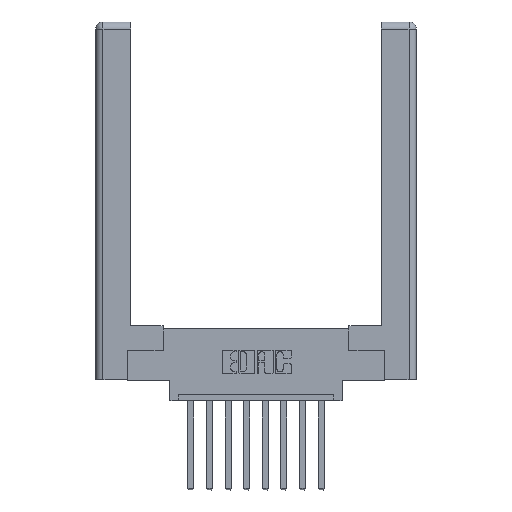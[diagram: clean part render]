
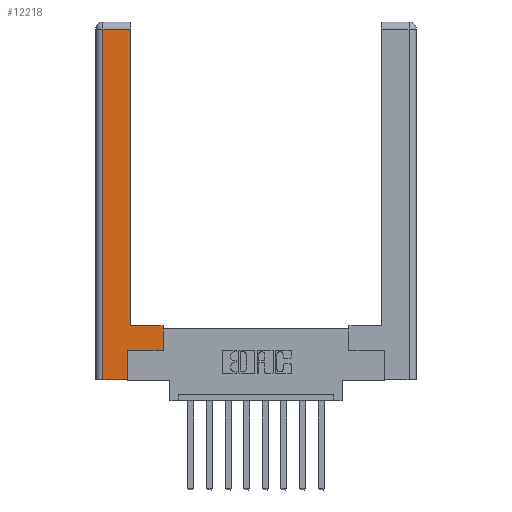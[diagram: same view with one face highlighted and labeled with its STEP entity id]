
A CAD part, top view. The second image highlights one B-rep face of the part: STEP entity #12218.
In plain terms, the highlighted planar face has unit normal (0, 0, 1).
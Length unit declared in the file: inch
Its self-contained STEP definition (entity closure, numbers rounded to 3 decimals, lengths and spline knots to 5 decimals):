
#433 = VECTOR ( 'NONE', #1633, 39.37008 ) ;
#869 = CARTESIAN_POINT ( 'NONE',  ( 0.0615, 0., 0. ) ) ;
#966 = EDGE_CURVE ( 'NONE', #11788, #7582, #6455, .T. ) ;
#1075 = VERTEX_POINT ( 'NONE', #1980 ) ;
#1281 = ORIENTED_EDGE ( 'NONE', *, *, #966, .T. ) ;
#1303 = LINE ( 'NONE', #11861, #8903 ) ;
#1392 = ORIENTED_EDGE ( 'NONE', *, *, #4505, .T. ) ;
#1480 = VERTEX_POINT ( 'NONE', #1637 ) ;
#1566 = DIRECTION ( 'NONE',  ( 0., 0., -1. ) ) ;
#1633 = DIRECTION ( 'NONE',  ( 0., 1., 0. ) ) ;
#1637 = CARTESIAN_POINT ( 'NONE',  ( 0.265, 0., 0. ) ) ;
#1784 = CARTESIAN_POINT ( 'NONE',  ( 0.0615, 2.94, 0. ) ) ;
#1980 = CARTESIAN_POINT ( 'NONE',  ( 0.295, 2.94, 0. ) ) ;
#1983 = CARTESIAN_POINT ( 'NONE',  ( 0.0615, 2.94, 0. ) ) ;
#2356 = VECTOR ( 'NONE', #12148, 39.37008 ) ;
#2391 = VECTOR ( 'NONE', #6361, 39.37008 ) ;
#3128 = ORIENTED_EDGE ( 'NONE', *, *, #3938, .T. ) ;
#3325 = CARTESIAN_POINT ( 'NONE',  ( 0.0615, 0., 0. ) ) ;
#3398 = EDGE_CURVE ( 'NONE', #7102, #9427, #4994, .T. ) ;
#3892 = EDGE_LOOP ( 'NONE', ( #7756, #9481, #7665, #5040, #1392, #8827, #1281, #3128 ) ) ;
#3938 = EDGE_CURVE ( 'NONE', #7582, #7434, #1303, .T. ) ;
#4505 = EDGE_CURVE ( 'NONE', #1480, #7061, #8411, .T. ) ;
#4525 = VECTOR ( 'NONE', #9711, 39.37008 ) ;
#4555 = EDGE_CURVE ( 'NONE', #7434, #1075, #5732, .T. ) ;
#4728 = LINE ( 'NONE', #1784, #4525 ) ;
#4894 = EDGE_CURVE ( 'NONE', #7061, #11788, #6653, .T. ) ;
#4994 = LINE ( 'NONE', #3325, #2391 ) ;
#5040 = ORIENTED_EDGE ( 'NONE', *, *, #11022, .T. ) ;
#5441 = CARTESIAN_POINT ( 'NONE',  ( 0.565, 0.245, 0. ) ) ;
#5732 = LINE ( 'NONE', #6259, #2356 ) ;
#5892 = DIRECTION ( 'NONE',  ( 1., 0., 0. ) ) ;
#6081 = EDGE_CURVE ( 'NONE', #1075, #7102, #4728, .T. ) ;
#6259 = CARTESIAN_POINT ( 'NONE',  ( 0.295, 3., 0. ) ) ;
#6361 = DIRECTION ( 'NONE',  ( 0., -1., 0. ) ) ;
#6382 = CARTESIAN_POINT ( 'NONE',  ( 0.265, 0., 0. ) ) ;
#6455 = LINE ( 'NONE', #7553, #433 ) ;
#6653 = LINE ( 'NONE', #10862, #11082 ) ;
#6964 = CARTESIAN_POINT ( 'NONE',  ( 0.265, 0.245, 0. ) ) ;
#7061 = VERTEX_POINT ( 'NONE', #6964 ) ;
#7096 = CARTESIAN_POINT ( 'NONE',  ( 0.265, 0.245, 0. ) ) ;
#7102 = VERTEX_POINT ( 'NONE', #1983 ) ;
#7331 = CARTESIAN_POINT ( 'NONE',  ( 0.565, 0.45, 0. ) ) ;
#7434 = VERTEX_POINT ( 'NONE', #9195 ) ;
#7453 = VECTOR ( 'NONE', #9136, 39.37008 ) ;
#7553 = CARTESIAN_POINT ( 'NONE',  ( 0.565, 0.45, 0. ) ) ;
#7582 = VERTEX_POINT ( 'NONE', #7331 ) ;
#7665 = ORIENTED_EDGE ( 'NONE', *, *, #3398, .T. ) ;
#7756 = ORIENTED_EDGE ( 'NONE', *, *, #4555, .T. ) ;
#8288 = CARTESIAN_POINT ( 'NONE',  ( 0., 0., 0. ) ) ;
#8411 = LINE ( 'NONE', #7096, #7453 ) ;
#8827 = ORIENTED_EDGE ( 'NONE', *, *, #4894, .T. ) ;
#8903 = VECTOR ( 'NONE', #9621, 39.37008 ) ;
#9136 = DIRECTION ( 'NONE',  ( 0., 1., 0. ) ) ;
#9195 = CARTESIAN_POINT ( 'NONE',  ( 0.295, 0.45, 0. ) ) ;
#9427 = VERTEX_POINT ( 'NONE', #869 ) ;
#9481 = ORIENTED_EDGE ( 'NONE', *, *, #6081, .T. ) ;
#9621 = DIRECTION ( 'NONE',  ( -1., 0., 0. ) ) ;
#9625 = VECTOR ( 'NONE', #5892, 39.37008 ) ;
#9711 = DIRECTION ( 'NONE',  ( -1., 0., 0. ) ) ;
#10111 = LINE ( 'NONE', #6382, #9625 ) ;
#10402 = DIRECTION ( 'NONE',  ( -1., 0., 0. ) ) ;
#10569 = FACE_OUTER_BOUND ( 'NONE', #3892, .T. ) ;
#10719 = AXIS2_PLACEMENT_3D ( 'NONE', #8288, #1566, #10402 ) ;
#10862 = CARTESIAN_POINT ( 'NONE',  ( 0.565, 0.245, 0. ) ) ;
#11022 = EDGE_CURVE ( 'NONE', #9427, #1480, #10111, .T. ) ;
#11082 = VECTOR ( 'NONE', #12915, 39.37008 ) ;
#11788 = VERTEX_POINT ( 'NONE', #5441 ) ;
#11861 = CARTESIAN_POINT ( 'NONE',  ( 0.295, 0.45, 0. ) ) ;
#12148 = DIRECTION ( 'NONE',  ( 0., 1., 0. ) ) ;
#12182 = PLANE ( 'NONE',  #10719 ) ;
#12218 = ADVANCED_FACE ( 'NONE', ( #10569 ), #12182, .F. ) ;
#12915 = DIRECTION ( 'NONE',  ( 1., 0., 0. ) ) ;
